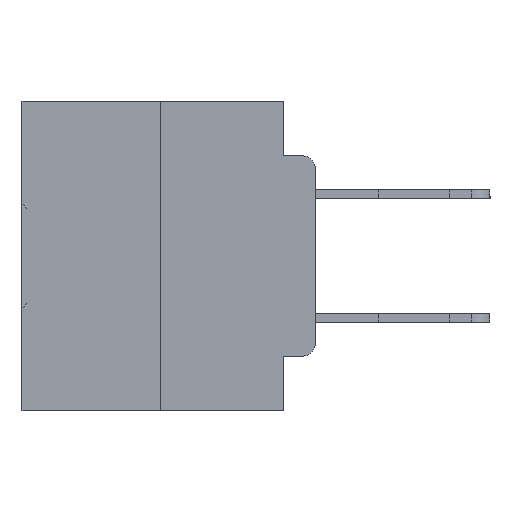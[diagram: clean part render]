
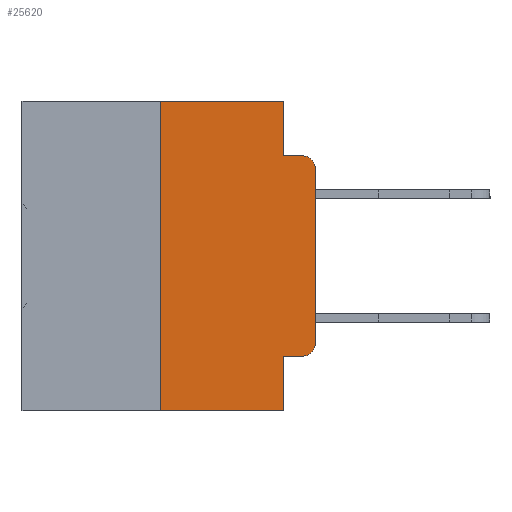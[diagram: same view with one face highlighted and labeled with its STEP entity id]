
A CAD part, left-side view. The second image highlights one B-rep face of the part: STEP entity #25620.
In plain terms, the highlighted planar face has unit normal (-1, 0, 0).
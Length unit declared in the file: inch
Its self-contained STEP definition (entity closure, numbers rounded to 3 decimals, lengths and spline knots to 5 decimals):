
#68 = VERTEX_POINT ( 'NONE', #18781 ) ;
#346 = VERTEX_POINT ( 'NONE', #30949 ) ;
#435 = VERTEX_POINT ( 'NONE', #30844 ) ;
#558 = ORIENTED_EDGE ( 'NONE', *, *, #32276, .F. ) ;
#783 = AXIS2_PLACEMENT_3D ( 'NONE', #27471, #851, #14505 ) ;
#851 = DIRECTION ( 'NONE',  ( 1., 0., 0. ) ) ;
#986 = DIRECTION ( 'NONE',  ( 0., -1., 0. ) ) ;
#1730 = VERTEX_POINT ( 'NONE', #27884 ) ;
#3702 = EDGE_CURVE ( 'NONE', #1730, #435, #13797, .T. ) ;
#4671 = CIRCLE ( 'NONE', #6820, 0.02 ) ;
#6272 = EDGE_CURVE ( 'NONE', #8085, #31504, #33110, .T. ) ;
#6549 = CARTESIAN_POINT ( 'NONE',  ( 0., 0.051, -0.0885 ) ) ;
#6586 = EDGE_CURVE ( 'NONE', #26736, #1730, #12733, .T. ) ;
#6598 = DIRECTION ( 'NONE',  ( 0., 0., 1. ) ) ;
#6736 = EDGE_LOOP ( 'NONE', ( #21418, #13586, #20840, #558, #18135, #10459, #16235, #14194, #20646, #12666 ) ) ;
#6820 = AXIS2_PLACEMENT_3D ( 'NONE', #13289, #31497, #15956 ) ;
#8085 = VERTEX_POINT ( 'NONE', #11062 ) ;
#8457 = DIRECTION ( 'NONE',  ( 0., -1., 0. ) ) ;
#9180 = CARTESIAN_POINT ( 'NONE',  ( 0., 0.473, 0. ) ) ;
#9254 = DIRECTION ( 'NONE',  ( 0., -1., 0. ) ) ;
#9484 = VECTOR ( 'NONE', #22637, 39.37008 ) ;
#9945 = LINE ( 'NONE', #9180, #30085 ) ;
#10459 = ORIENTED_EDGE ( 'NONE', *, *, #6272, .F. ) ;
#10549 = CARTESIAN_POINT ( 'NONE',  ( 0., 0.473, -0.5 ) ) ;
#11062 = CARTESIAN_POINT ( 'NONE',  ( 0., 0.25, -0.5 ) ) ;
#12666 = ORIENTED_EDGE ( 'NONE', *, *, #6586, .T. ) ;
#12733 = CIRCLE ( 'NONE', #30193, 0.02 ) ;
#13020 = CARTESIAN_POINT ( 'NONE',  ( 0., 0.051, 0. ) ) ;
#13289 = CARTESIAN_POINT ( 'NONE',  ( 0., 0.02, -0.1085 ) ) ;
#13317 = DIRECTION ( 'NONE',  ( -1., 0., 0. ) ) ;
#13586 = ORIENTED_EDGE ( 'NONE', *, *, #23107, .T. ) ;
#13727 = VECTOR ( 'NONE', #9254, 39.37008 ) ;
#13797 = LINE ( 'NONE', #22089, #14626 ) ;
#14194 = ORIENTED_EDGE ( 'NONE', *, *, #18187, .F. ) ;
#14288 = VERTEX_POINT ( 'NONE', #34090 ) ;
#14505 = DIRECTION ( 'NONE',  ( 0., 0., -1. ) ) ;
#14626 = VECTOR ( 'NONE', #25805, 39.37008 ) ;
#14706 = CARTESIAN_POINT ( 'NONE',  ( 0., 0.051, 0. ) ) ;
#15956 = DIRECTION ( 'NONE',  ( 0., 0., -1. ) ) ;
#16235 = ORIENTED_EDGE ( 'NONE', *, *, #28248, .T. ) ;
#17947 = EDGE_CURVE ( 'NONE', #68, #26736, #20331, .T. ) ;
#18135 = ORIENTED_EDGE ( 'NONE', *, *, #31612, .F. ) ;
#18187 = EDGE_CURVE ( 'NONE', #68, #28289, #32884, .T. ) ;
#18225 = LINE ( 'NONE', #30500, #9484 ) ;
#18781 = CARTESIAN_POINT ( 'NONE',  ( 0., 0.051, -0.4115 ) ) ;
#18998 = EDGE_CURVE ( 'NONE', #14288, #346, #27578, .T. ) ;
#19187 = CARTESIAN_POINT ( 'NONE',  ( 0., 0.25, 0. ) ) ;
#20331 = LINE ( 'NONE', #24256, #28058 ) ;
#20646 = ORIENTED_EDGE ( 'NONE', *, *, #17947, .T. ) ;
#20840 = ORIENTED_EDGE ( 'NONE', *, *, #18998, .F. ) ;
#21174 = DIRECTION ( 'NONE',  ( 0., -1., 0. ) ) ;
#21418 = ORIENTED_EDGE ( 'NONE', *, *, #3702, .T. ) ;
#22089 = CARTESIAN_POINT ( 'NONE',  ( 0., 0., 0. ) ) ;
#22471 = CARTESIAN_POINT ( 'NONE',  ( 0., 0.25, 0. ) ) ;
#22637 = DIRECTION ( 'NONE',  ( 0., 0., -1. ) ) ;
#23107 = EDGE_CURVE ( 'NONE', #435, #346, #4671, .T. ) ;
#23872 = CARTESIAN_POINT ( 'NONE',  ( 0., 0.051, -0.5 ) ) ;
#24256 = CARTESIAN_POINT ( 'NONE',  ( 0., 0.051, -0.4115 ) ) ;
#24885 = CARTESIAN_POINT ( 'NONE',  ( 0., 0.02, -0.4115 ) ) ;
#25620 = ADVANCED_FACE ( 'NONE', ( #25741 ), #30092, .F. ) ;
#25741 = FACE_OUTER_BOUND ( 'NONE', #6736, .T. ) ;
#25805 = DIRECTION ( 'NONE',  ( 0., 0., 1. ) ) ;
#26213 = VECTOR ( 'NONE', #6598, 39.37008 ) ;
#26736 = VERTEX_POINT ( 'NONE', #24885 ) ;
#26819 = VECTOR ( 'NONE', #21174, 39.37008 ) ;
#27021 = VERTEX_POINT ( 'NONE', #13020 ) ;
#27471 = CARTESIAN_POINT ( 'NONE',  ( 0., 0.473, 0. ) ) ;
#27578 = LINE ( 'NONE', #6549, #13727 ) ;
#27664 = LINE ( 'NONE', #10549, #26819 ) ;
#27884 = CARTESIAN_POINT ( 'NONE',  ( 0., 0., -0.3915 ) ) ;
#28058 = VECTOR ( 'NONE', #8457, 39.37008 ) ;
#28248 = EDGE_CURVE ( 'NONE', #8085, #28289, #27664, .T. ) ;
#28289 = VERTEX_POINT ( 'NONE', #23872 ) ;
#28932 = CARTESIAN_POINT ( 'NONE',  ( 0., 0.02, -0.3915 ) ) ;
#30085 = VECTOR ( 'NONE', #986, 39.37008 ) ;
#30092 = PLANE ( 'NONE',  #783 ) ;
#30193 = AXIS2_PLACEMENT_3D ( 'NONE', #28932, #13317, #31525 ) ;
#30400 = DIRECTION ( 'NONE',  ( 0., 0., -1. ) ) ;
#30500 = CARTESIAN_POINT ( 'NONE',  ( 0., 0.051, 0. ) ) ;
#30844 = CARTESIAN_POINT ( 'NONE',  ( 0., 0., -0.1085 ) ) ;
#30949 = CARTESIAN_POINT ( 'NONE',  ( 0., 0.02, -0.0885 ) ) ;
#31497 = DIRECTION ( 'NONE',  ( -1., 0., 0. ) ) ;
#31504 = VERTEX_POINT ( 'NONE', #19187 ) ;
#31525 = DIRECTION ( 'NONE',  ( 0., 0., -1. ) ) ;
#31612 = EDGE_CURVE ( 'NONE', #31504, #27021, #9945, .T. ) ;
#32083 = VECTOR ( 'NONE', #30400, 39.37008 ) ;
#32276 = EDGE_CURVE ( 'NONE', #27021, #14288, #18225, .T. ) ;
#32884 = LINE ( 'NONE', #14706, #32083 ) ;
#33110 = LINE ( 'NONE', #22471, #26213 ) ;
#34090 = CARTESIAN_POINT ( 'NONE',  ( 0., 0.051, -0.0885 ) ) ;
